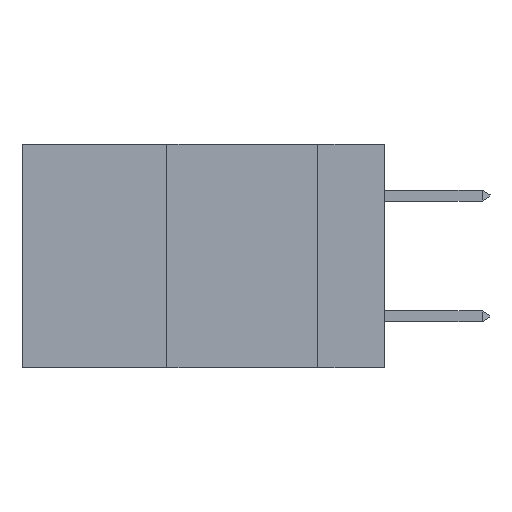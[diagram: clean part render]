
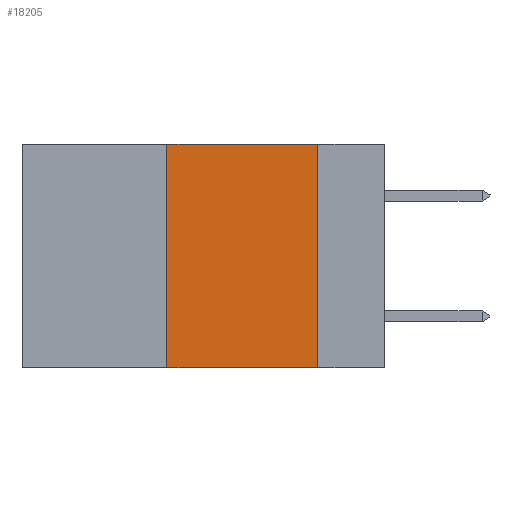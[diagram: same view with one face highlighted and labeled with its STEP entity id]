
A CAD part, left-side view. The second image highlights one B-rep face of the part: STEP entity #18205.
In plain terms, the highlighted planar face has unit normal (-1, 0, 0).
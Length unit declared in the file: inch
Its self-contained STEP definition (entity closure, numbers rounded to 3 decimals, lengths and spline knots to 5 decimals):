
#445 = EDGE_CURVE ( 'NONE', #24347, #10407, #8099, .T. ) ;
#521 = LINE ( 'NONE', #24559, #23633 ) ;
#648 = CARTESIAN_POINT ( 'NONE',  ( 0., 0.6, 0. ) ) ;
#676 = CARTESIAN_POINT ( 'NONE',  ( 0., 0.11, 0. ) ) ;
#987 = DIRECTION ( 'NONE',  ( 0., -1., 0. ) ) ;
#1806 = DIRECTION ( 'NONE',  ( 0., -1., 0. ) ) ;
#2477 = ORIENTED_EDGE ( 'NONE', *, *, #445, .T. ) ;
#4103 = EDGE_LOOP ( 'NONE', ( #9347, #27356, #11136, #2477 ) ) ;
#5334 = CARTESIAN_POINT ( 'NONE',  ( 0., 0.6, 0. ) ) ;
#5477 = CARTESIAN_POINT ( 'NONE',  ( 0., 0.6, -0.37 ) ) ;
#5778 = LINE ( 'NONE', #21766, #27469 ) ;
#8099 = LINE ( 'NONE', #5477, #11174 ) ;
#9347 = ORIENTED_EDGE ( 'NONE', *, *, #18915, .F. ) ;
#10407 = VERTEX_POINT ( 'NONE', #24596 ) ;
#10999 = LINE ( 'NONE', #5334, #14055 ) ;
#11136 = ORIENTED_EDGE ( 'NONE', *, *, #20046, .F. ) ;
#11174 = VECTOR ( 'NONE', #1806, 39.37008 ) ;
#12903 = VERTEX_POINT ( 'NONE', #15275 ) ;
#13764 = PLANE ( 'NONE',  #23591 ) ;
#14055 = VECTOR ( 'NONE', #987, 39.37008 ) ;
#15275 = CARTESIAN_POINT ( 'NONE',  ( 0., 0.36, 0. ) ) ;
#16145 = VERTEX_POINT ( 'NONE', #676 ) ;
#18164 = EDGE_CURVE ( 'NONE', #12903, #16145, #10999, .T. ) ;
#18205 = ADVANCED_FACE ( 'NONE', ( #25114 ), #13764, .F. ) ;
#18915 = EDGE_CURVE ( 'NONE', #16145, #10407, #5778, .T. ) ;
#20046 = EDGE_CURVE ( 'NONE', #24347, #12903, #521, .T. ) ;
#20595 = DIRECTION ( 'NONE',  ( 0., 0., -1. ) ) ;
#20788 = DIRECTION ( 'NONE',  ( 1., 0., 0. ) ) ;
#21766 = CARTESIAN_POINT ( 'NONE',  ( 0., 0.11, 0. ) ) ;
#22514 = DIRECTION ( 'NONE',  ( 0., 0., 1. ) ) ;
#23591 = AXIS2_PLACEMENT_3D ( 'NONE', #648, #20788, #20595 ) ;
#23633 = VECTOR ( 'NONE', #22514, 39.37008 ) ;
#23737 = CARTESIAN_POINT ( 'NONE',  ( 0., 0.36, -0.37 ) ) ;
#23970 = DIRECTION ( 'NONE',  ( 0., 0., -1. ) ) ;
#24347 = VERTEX_POINT ( 'NONE', #23737 ) ;
#24559 = CARTESIAN_POINT ( 'NONE',  ( 0., 0.36, 0. ) ) ;
#24596 = CARTESIAN_POINT ( 'NONE',  ( 0., 0.11, -0.37 ) ) ;
#25114 = FACE_OUTER_BOUND ( 'NONE', #4103, .T. ) ;
#27356 = ORIENTED_EDGE ( 'NONE', *, *, #18164, .F. ) ;
#27469 = VECTOR ( 'NONE', #23970, 39.37008 ) ;
